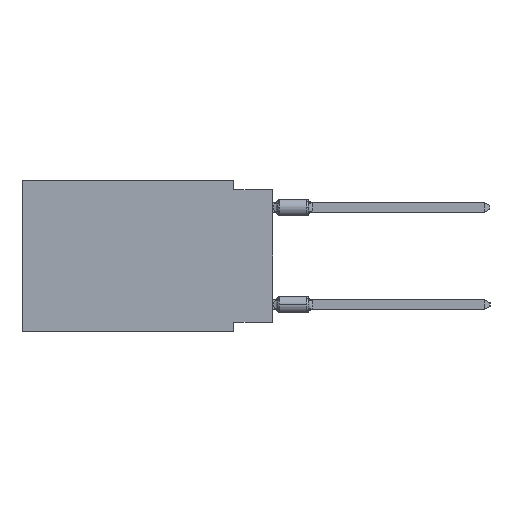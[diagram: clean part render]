
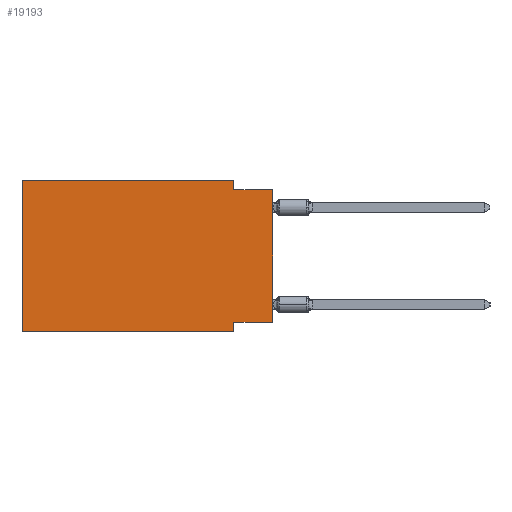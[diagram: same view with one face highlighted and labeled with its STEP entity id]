
A CAD part, left-side view. The second image highlights one B-rep face of the part: STEP entity #19193.
In plain terms, the highlighted planar face has unit normal (-1, 0, 0).
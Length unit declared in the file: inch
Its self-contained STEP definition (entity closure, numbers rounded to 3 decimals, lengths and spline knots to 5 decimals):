
#1071 = VECTOR ( 'NONE', #46716, 39.37008 ) ;
#1138 = CARTESIAN_POINT ( 'NONE',  ( 0., 0.1, -0.025 ) ) ;
#1773 = DIRECTION ( 'NONE',  ( 0., 0., 1. ) ) ;
#1876 = VECTOR ( 'NONE', #45326, 39.37008 ) ;
#2497 = EDGE_CURVE ( 'NONE', #33374, #16343, #47280, .T. ) ;
#2504 = VERTEX_POINT ( 'NONE', #3693 ) ;
#3693 = CARTESIAN_POINT ( 'NONE',  ( 0., 0., -0.365 ) ) ;
#4108 = LINE ( 'NONE', #22783, #1876 ) ;
#4469 = EDGE_LOOP ( 'NONE', ( #38935, #36263, #16248, #44908, #45279, #10799, #51739, #20442 ) ) ;
#6087 = EDGE_CURVE ( 'NONE', #2504, #33374, #33433, .T. ) ;
#6691 = EDGE_CURVE ( 'NONE', #2504, #8527, #4108, .T. ) ;
#8527 = VERTEX_POINT ( 'NONE', #45261 ) ;
#8880 = CARTESIAN_POINT ( 'NONE',  ( 0., 0., -0.025 ) ) ;
#10387 = VERTEX_POINT ( 'NONE', #39836 ) ;
#10799 = ORIENTED_EDGE ( 'NONE', *, *, #12741, .T. ) ;
#11226 = DIRECTION ( 'NONE',  ( 0., 1., 0. ) ) ;
#12741 = EDGE_CURVE ( 'NONE', #10387, #16343, #51070, .T. ) ;
#13338 = EDGE_CURVE ( 'NONE', #26430, #52899, #20819, .T. ) ;
#13416 = DIRECTION ( 'NONE',  ( 0., 0., -1. ) ) ;
#15625 = CARTESIAN_POINT ( 'NONE',  ( 0., 0.1, 0. ) ) ;
#16135 = CARTESIAN_POINT ( 'NONE',  ( 0., 0.645, 0. ) ) ;
#16248 = ORIENTED_EDGE ( 'NONE', *, *, #53287, .F. ) ;
#16343 = VERTEX_POINT ( 'NONE', #39544 ) ;
#16379 = VECTOR ( 'NONE', #40441, 39.37008 ) ;
#18860 = EDGE_CURVE ( 'NONE', #24085, #8527, #48682, .T. ) ;
#19193 = ADVANCED_FACE ( 'NONE', ( #43055 ), #26576, .F. ) ;
#20442 = ORIENTED_EDGE ( 'NONE', *, *, #6087, .F. ) ;
#20572 = EDGE_CURVE ( 'NONE', #10387, #26430, #40974, .T. ) ;
#20819 = LINE ( 'NONE', #16135, #53389 ) ;
#20932 = CARTESIAN_POINT ( 'NONE',  ( 0., 0.1, -0.39 ) ) ;
#21742 = VECTOR ( 'NONE', #39059, 39.37008 ) ;
#22783 = CARTESIAN_POINT ( 'NONE',  ( 0., 0., 0. ) ) ;
#22920 = VECTOR ( 'NONE', #1773, 39.37008 ) ;
#23680 = CARTESIAN_POINT ( 'NONE',  ( 0., 0.645, 0. ) ) ;
#24085 = VERTEX_POINT ( 'NONE', #1138 ) ;
#26430 = VERTEX_POINT ( 'NONE', #23680 ) ;
#26576 = PLANE ( 'NONE',  #38844 ) ;
#27865 = VECTOR ( 'NONE', #55698, 39.37008 ) ;
#29077 = LINE ( 'NONE', #15625, #27865 ) ;
#33374 = VERTEX_POINT ( 'NONE', #54924 ) ;
#33433 = LINE ( 'NONE', #51273, #54155 ) ;
#36263 = ORIENTED_EDGE ( 'NONE', *, *, #18860, .F. ) ;
#37502 = CARTESIAN_POINT ( 'NONE',  ( 0., 0.645, 0. ) ) ;
#38844 = AXIS2_PLACEMENT_3D ( 'NONE', #37502, #53485, #13416 ) ;
#38935 = ORIENTED_EDGE ( 'NONE', *, *, #6691, .T. ) ;
#39059 = DIRECTION ( 'NONE',  ( 0., 0., -1. ) ) ;
#39544 = CARTESIAN_POINT ( 'NONE',  ( 0., 0.1, -0.39 ) ) ;
#39836 = CARTESIAN_POINT ( 'NONE',  ( 0., 0.645, -0.39 ) ) ;
#40441 = DIRECTION ( 'NONE',  ( 0., -1., 0. ) ) ;
#40974 = LINE ( 'NONE', #41854, #22920 ) ;
#41854 = CARTESIAN_POINT ( 'NONE',  ( 0., 0.645, 0. ) ) ;
#42394 = CARTESIAN_POINT ( 'NONE',  ( 0., 0.1, 0. ) ) ;
#43055 = FACE_OUTER_BOUND ( 'NONE', #4469, .T. ) ;
#44908 = ORIENTED_EDGE ( 'NONE', *, *, #13338, .F. ) ;
#45261 = CARTESIAN_POINT ( 'NONE',  ( 0., 0., -0.025 ) ) ;
#45279 = ORIENTED_EDGE ( 'NONE', *, *, #20572, .F. ) ;
#45326 = DIRECTION ( 'NONE',  ( 0., 0., 1. ) ) ;
#46716 = DIRECTION ( 'NONE',  ( 0., -1., 0. ) ) ;
#47280 = LINE ( 'NONE', #20932, #21742 ) ;
#48682 = LINE ( 'NONE', #8880, #16379 ) ;
#51070 = LINE ( 'NONE', #51358, #1071 ) ;
#51273 = CARTESIAN_POINT ( 'NONE',  ( 0., 0., -0.365 ) ) ;
#51358 = CARTESIAN_POINT ( 'NONE',  ( 0., 0.645, -0.39 ) ) ;
#51739 = ORIENTED_EDGE ( 'NONE', *, *, #2497, .F. ) ;
#52899 = VERTEX_POINT ( 'NONE', #42394 ) ;
#53287 = EDGE_CURVE ( 'NONE', #52899, #24085, #29077, .T. ) ;
#53389 = VECTOR ( 'NONE', #56489, 39.37008 ) ;
#53485 = DIRECTION ( 'NONE',  ( 1., 0., 0. ) ) ;
#54155 = VECTOR ( 'NONE', #11226, 39.37008 ) ;
#54924 = CARTESIAN_POINT ( 'NONE',  ( 0., 0.1, -0.365 ) ) ;
#55698 = DIRECTION ( 'NONE',  ( 0., 0., -1. ) ) ;
#56489 = DIRECTION ( 'NONE',  ( 0., -1., 0. ) ) ;
